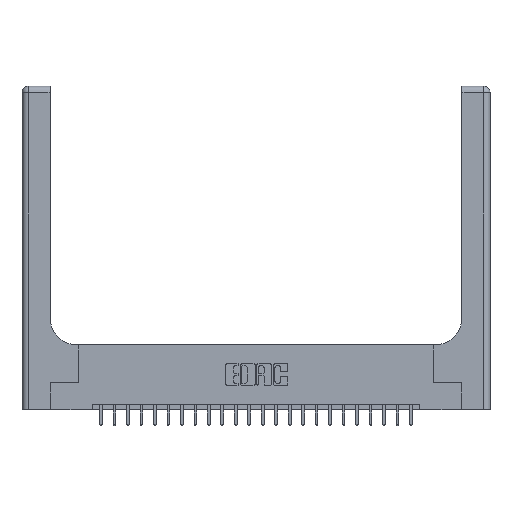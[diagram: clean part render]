
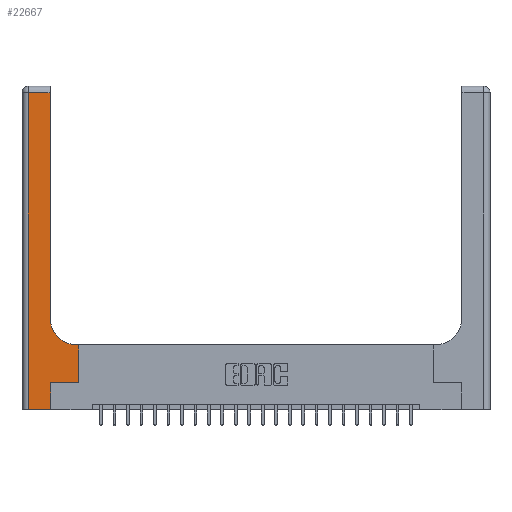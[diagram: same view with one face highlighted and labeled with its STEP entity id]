
A CAD part, top view. The second image highlights one B-rep face of the part: STEP entity #22667.
In plain terms, the highlighted planar face has unit normal (0, 0, 1).
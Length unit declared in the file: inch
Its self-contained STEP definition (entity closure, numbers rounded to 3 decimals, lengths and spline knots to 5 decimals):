
#230 = ORIENTED_EDGE ( 'NONE', *, *, #22987, .T. ) ;
#645 = VERTEX_POINT ( 'NONE', #776 ) ;
#667 = LINE ( 'NONE', #7509, #18772 ) ;
#775 = CARTESIAN_POINT ( 'NONE',  ( 0.265, 0., 0.37 ) ) ;
#776 = CARTESIAN_POINT ( 'NONE',  ( 0.06, 0., 0.37 ) ) ;
#1186 = VECTOR ( 'NONE', #18863, 39.37008 ) ;
#1343 = EDGE_CURVE ( 'NONE', #6284, #9672, #5274, .T. ) ;
#1806 = CARTESIAN_POINT ( 'NONE',  ( 0., 0., 0.37 ) ) ;
#2247 = CARTESIAN_POINT ( 'NONE',  ( 0.528, 0.6, 0.37 ) ) ;
#2584 = CARTESIAN_POINT ( 'NONE',  ( 0.06, 3., 0.37 ) ) ;
#2735 = LINE ( 'NONE', #17253, #16718 ) ;
#3164 = ORIENTED_EDGE ( 'NONE', *, *, #1343, .T. ) ;
#3165 = VECTOR ( 'NONE', #18909, 39.37008 ) ;
#3231 = DIRECTION ( 'NONE',  ( 1., 0., 0. ) ) ;
#3346 = CARTESIAN_POINT ( 'NONE',  ( 0.265, 0.25, 0.37 ) ) ;
#3447 = EDGE_CURVE ( 'NONE', #11076, #15145, #22243, .T. ) ;
#3943 = DIRECTION ( 'NONE',  ( 0., 1., 0. ) ) ;
#4237 = CARTESIAN_POINT ( 'NONE',  ( 0.26, 3., 0.37 ) ) ;
#4466 = ORIENTED_EDGE ( 'NONE', *, *, #20025, .T. ) ;
#5274 = LINE ( 'NONE', #3346, #19068 ) ;
#5719 = LINE ( 'NONE', #2584, #3165 ) ;
#6284 = VERTEX_POINT ( 'NONE', #14468 ) ;
#6517 = AXIS2_PLACEMENT_3D ( 'NONE', #8832, #14484, #16393 ) ;
#7509 = CARTESIAN_POINT ( 'NONE',  ( 0.265, 0., 0.37 ) ) ;
#7665 = CIRCLE ( 'NONE', #6517, 0.25 ) ;
#7688 = FACE_OUTER_BOUND ( 'NONE', #23656, .T. ) ;
#7880 = ORIENTED_EDGE ( 'NONE', *, *, #8980, .T. ) ;
#8832 = CARTESIAN_POINT ( 'NONE',  ( 0.51, 0.85, 0.37 ) ) ;
#8980 = EDGE_CURVE ( 'NONE', #645, #11928, #9003, .T. ) ;
#9003 = LINE ( 'NONE', #1806, #21506 ) ;
#9027 = LINE ( 'NONE', #23471, #14940 ) ;
#9672 = VERTEX_POINT ( 'NONE', #23002 ) ;
#9682 = LINE ( 'NONE', #12939, #17208 ) ;
#9776 = ORIENTED_EDGE ( 'NONE', *, *, #20736, .T. ) ;
#10643 = CARTESIAN_POINT ( 'NONE',  ( 0.26, 0.85, 0.37 ) ) ;
#11076 = VERTEX_POINT ( 'NONE', #10643 ) ;
#11174 = DIRECTION ( 'NONE',  ( -1., 0., 0. ) ) ;
#11261 = EDGE_CURVE ( 'NONE', #19889, #645, #5719, .T. ) ;
#11616 = DIRECTION ( 'NONE',  ( -1., 0., 0. ) ) ;
#11928 = VERTEX_POINT ( 'NONE', #775 ) ;
#12181 = DIRECTION ( 'NONE',  ( -1., 0., 0. ) ) ;
#12863 = CARTESIAN_POINT ( 'NONE',  ( 0., 3., 0.37 ) ) ;
#12939 = CARTESIAN_POINT ( 'NONE',  ( 0.528, 0.25, 0.37 ) ) ;
#13509 = DIRECTION ( 'NONE',  ( 0., 1., 0. ) ) ;
#14468 = CARTESIAN_POINT ( 'NONE',  ( 0.265, 0.25, 0.37 ) ) ;
#14484 = DIRECTION ( 'NONE',  ( 0., 0., -1. ) ) ;
#14940 = VECTOR ( 'NONE', #12181, 39.37008 ) ;
#15145 = VERTEX_POINT ( 'NONE', #16453 ) ;
#15848 = VERTEX_POINT ( 'NONE', #2247 ) ;
#16178 = ORIENTED_EDGE ( 'NONE', *, *, #3447, .T. ) ;
#16393 = DIRECTION ( 'NONE',  ( 1., 0., 0. ) ) ;
#16453 = CARTESIAN_POINT ( 'NONE',  ( 0.26, 2.94, 0.37 ) ) ;
#16718 = VECTOR ( 'NONE', #11616, 39.37008 ) ;
#16946 = ORIENTED_EDGE ( 'NONE', *, *, #11261, .T. ) ;
#17205 = EDGE_CURVE ( 'NONE', #15848, #19807, #2735, .T. ) ;
#17208 = VECTOR ( 'NONE', #3943, 39.37008 ) ;
#17253 = CARTESIAN_POINT ( 'NONE',  ( 0.26, 0.6, 0.37 ) ) ;
#17895 = DIRECTION ( 'NONE',  ( 1., 0., 0. ) ) ;
#18105 = CARTESIAN_POINT ( 'NONE',  ( 0.06, 2.94, 0.37 ) ) ;
#18772 = VECTOR ( 'NONE', #13509, 39.37008 ) ;
#18863 = DIRECTION ( 'NONE',  ( 0., 1., 0. ) ) ;
#18909 = DIRECTION ( 'NONE',  ( 0., -1., 0. ) ) ;
#19068 = VECTOR ( 'NONE', #3231, 39.37008 ) ;
#19206 = CARTESIAN_POINT ( 'NONE',  ( 0.51, 0.6, 0.37 ) ) ;
#19807 = VERTEX_POINT ( 'NONE', #19206 ) ;
#19889 = VERTEX_POINT ( 'NONE', #18105 ) ;
#20025 = EDGE_CURVE ( 'NONE', #9672, #15848, #9682, .T. ) ;
#20183 = DIRECTION ( 'NONE',  ( 0., 0., -1. ) ) ;
#20691 = ORIENTED_EDGE ( 'NONE', *, *, #21587, .T. ) ;
#20735 = AXIS2_PLACEMENT_3D ( 'NONE', #12863, #20183, #11174 ) ;
#20736 = EDGE_CURVE ( 'NONE', #15145, #19889, #9027, .T. ) ;
#21506 = VECTOR ( 'NONE', #17895, 39.37008 ) ;
#21587 = EDGE_CURVE ( 'NONE', #19807, #11076, #7665, .T. ) ;
#21984 = PLANE ( 'NONE',  #20735 ) ;
#22243 = LINE ( 'NONE', #4237, #1186 ) ;
#22667 = ADVANCED_FACE ( 'NONE', ( #7688 ), #21984, .F. ) ;
#22776 = ORIENTED_EDGE ( 'NONE', *, *, #17205, .T. ) ;
#22987 = EDGE_CURVE ( 'NONE', #11928, #6284, #667, .T. ) ;
#23002 = CARTESIAN_POINT ( 'NONE',  ( 0.528, 0.25, 0.37 ) ) ;
#23471 = CARTESIAN_POINT ( 'NONE',  ( 0., 2.94, 0.37 ) ) ;
#23656 = EDGE_LOOP ( 'NONE', ( #16178, #9776, #16946, #7880, #230, #3164, #4466, #22776, #20691 ) ) ;
